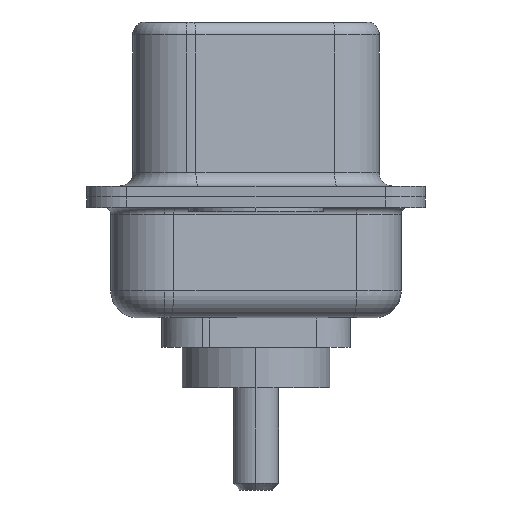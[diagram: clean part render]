
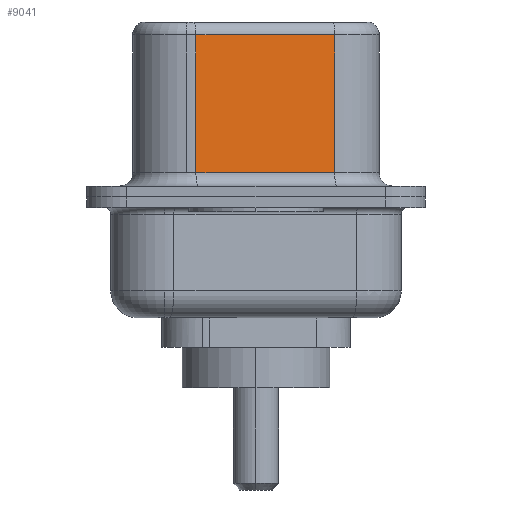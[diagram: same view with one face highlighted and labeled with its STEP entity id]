
A CAD part, left-side view. The second image highlights one B-rep face of the part: STEP entity #9041.
In plain terms, the highlighted planar face has unit normal (-0.985, -0.174, 0).
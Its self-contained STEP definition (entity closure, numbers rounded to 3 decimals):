
#797 = EDGE_LOOP ( 'NONE', ( #4562, #7206, #10773, #2914 ) ) ;
#825 = EDGE_CURVE ( 'NONE', #1799, #8132, #8209, .T. ) ;
#1108 = EDGE_CURVE ( 'NONE', #8132, #7308, #7514, .T. ) ;
#1353 = VECTOR ( 'NONE', #9763, 1000. ) ;
#1475 = DIRECTION ( 'NONE',  ( 0., 0., -1. ) ) ;
#1551 = EDGE_CURVE ( 'NONE', #1799, #8547, #7793, .T. ) ;
#1799 = VERTEX_POINT ( 'NONE', #10531 ) ;
#2812 = CARTESIAN_POINT ( 'NONE',  ( 3.655, 2.233, 6.02 ) ) ;
#2843 = PLANE ( 'NONE',  #9155 ) ;
#2914 = ORIENTED_EDGE ( 'NONE', *, *, #8499, .T. ) ;
#2936 = DIRECTION ( 'NONE',  ( 0.174, -0.985, 0. ) ) ;
#3160 = CARTESIAN_POINT ( 'NONE',  ( 3.655, 2.233, 6.52 ) ) ;
#3913 = CARTESIAN_POINT ( 'NONE',  ( 4.565, -2.927, 0.9 ) ) ;
#4562 = ORIENTED_EDGE ( 'NONE', *, *, #1551, .F. ) ;
#5262 = VECTOR ( 'NONE', #1475, 1000. ) ;
#5576 = CARTESIAN_POINT ( 'NONE',  ( 4.565, -2.927, 6.52 ) ) ;
#5918 = VECTOR ( 'NONE', #6542, 1000. ) ;
#6542 = DIRECTION ( 'NONE',  ( -0.174, 0.985, 0. ) ) ;
#6548 = CARTESIAN_POINT ( 'NONE',  ( 3.655, 2.233, 0.9 ) ) ;
#6566 = VECTOR ( 'NONE', #2936, 1000. ) ;
#7206 = ORIENTED_EDGE ( 'NONE', *, *, #825, .T. ) ;
#7308 = VERTEX_POINT ( 'NONE', #6548 ) ;
#7514 = LINE ( 'NONE', #3160, #5262 ) ;
#7793 = LINE ( 'NONE', #5576, #1353 ) ;
#8132 = VERTEX_POINT ( 'NONE', #2812 ) ;
#8140 = CARTESIAN_POINT ( 'NONE',  ( 4.565, -2.927, 6.52 ) ) ;
#8209 = LINE ( 'NONE', #8332, #5918 ) ;
#8332 = CARTESIAN_POINT ( 'NONE',  ( 4.565, -2.927, 6.02 ) ) ;
#8499 = EDGE_CURVE ( 'NONE', #7308, #8547, #9118, .T. ) ;
#8547 = VERTEX_POINT ( 'NONE', #3913 ) ;
#9041 = ADVANCED_FACE ( 'NONE', ( #10350 ), #2843, .F. ) ;
#9118 = LINE ( 'NONE', #10448, #6566 ) ;
#9155 = AXIS2_PLACEMENT_3D ( 'NONE', #8140, #9553, #9361 ) ;
#9361 = DIRECTION ( 'NONE',  ( -0.174, 0.985, 0. ) ) ;
#9553 = DIRECTION ( 'NONE',  ( 0.985, 0.174, 0. ) ) ;
#9763 = DIRECTION ( 'NONE',  ( 0., 0., -1. ) ) ;
#10350 = FACE_OUTER_BOUND ( 'NONE', #797, .T. ) ;
#10448 = CARTESIAN_POINT ( 'NONE',  ( 4.565, -2.927, 0.9 ) ) ;
#10531 = CARTESIAN_POINT ( 'NONE',  ( 4.565, -2.927, 6.02 ) ) ;
#10773 = ORIENTED_EDGE ( 'NONE', *, *, #1108, .T. ) ;
